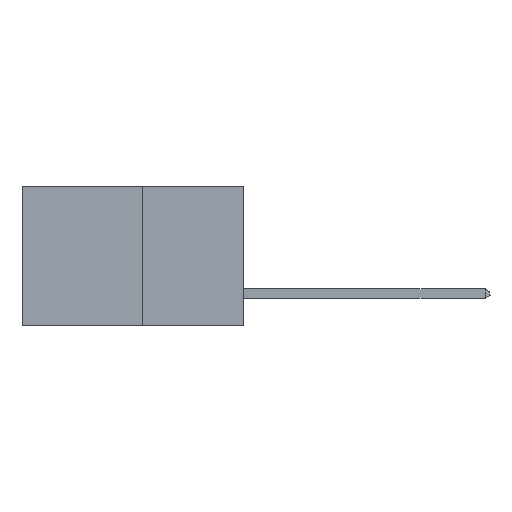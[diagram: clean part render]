
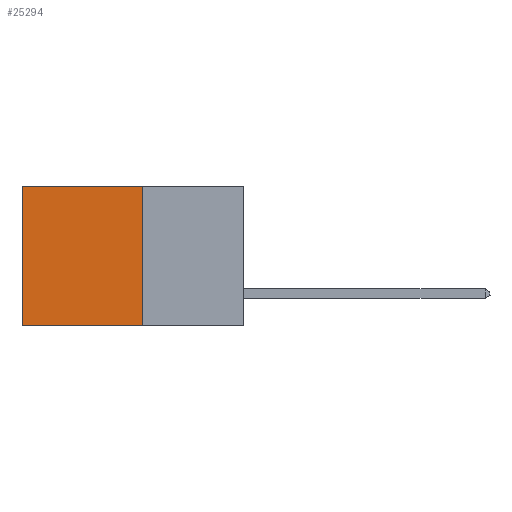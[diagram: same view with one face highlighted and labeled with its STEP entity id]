
A CAD part, left-side view. The second image highlights one B-rep face of the part: STEP entity #25294.
In plain terms, the highlighted planar face has unit normal (-1, 0, 0).
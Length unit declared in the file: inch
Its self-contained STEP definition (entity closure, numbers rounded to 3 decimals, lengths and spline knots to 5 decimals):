
#640 = CARTESIAN_POINT ( 'NONE',  ( 0.277, 0.59, 0. ) ) ;
#789 = DIRECTION ( 'NONE',  ( 0., 1., 0. ) ) ;
#1320 = VERTEX_POINT ( 'NONE', #11204 ) ;
#1961 = CARTESIAN_POINT ( 'NONE',  ( 0.277, 0.27, -0.37 ) ) ;
#2572 = EDGE_CURVE ( 'NONE', #13739, #1320, #28361, .T. ) ;
#3991 = VECTOR ( 'NONE', #12583, 39.37008 ) ;
#4386 = FACE_OUTER_BOUND ( 'NONE', #16905, .T. ) ;
#5601 = ORIENTED_EDGE ( 'NONE', *, *, #12651, .F. ) ;
#6163 = AXIS2_PLACEMENT_3D ( 'NONE', #1961, #22566, #9011 ) ;
#6635 = LINE ( 'NONE', #16857, #12739 ) ;
#6698 = PLANE ( 'NONE',  #6163 ) ;
#9011 = DIRECTION ( 'NONE',  ( 0., 0., -1. ) ) ;
#10261 = VERTEX_POINT ( 'NONE', #640 ) ;
#10298 = CARTESIAN_POINT ( 'NONE',  ( 0.277, 0.59, -0.37 ) ) ;
#10349 = EDGE_CURVE ( 'NONE', #10261, #1320, #22900, .T. ) ;
#10767 = VERTEX_POINT ( 'NONE', #20615 ) ;
#11204 = CARTESIAN_POINT ( 'NONE',  ( 0.277, 0.59, -0.37 ) ) ;
#12583 = DIRECTION ( 'NONE',  ( 0., 0., -1. ) ) ;
#12651 = EDGE_CURVE ( 'NONE', #10767, #13739, #23096, .T. ) ;
#12739 = VECTOR ( 'NONE', #789, 39.37008 ) ;
#13739 = VERTEX_POINT ( 'NONE', #24845 ) ;
#14686 = DIRECTION ( 'NONE',  ( 0., 0., -1. ) ) ;
#16041 = ORIENTED_EDGE ( 'NONE', *, *, #10349, .T. ) ;
#16857 = CARTESIAN_POINT ( 'NONE',  ( 0.277, 0.27, 0. ) ) ;
#16905 = EDGE_LOOP ( 'NONE', ( #16041, #18415, #5601, #23779 ) ) ;
#18415 = ORIENTED_EDGE ( 'NONE', *, *, #2572, .F. ) ;
#19238 = EDGE_CURVE ( 'NONE', #10767, #10261, #6635, .T. ) ;
#20615 = CARTESIAN_POINT ( 'NONE',  ( 0.277, 0.27, 0. ) ) ;
#21403 = CARTESIAN_POINT ( 'NONE',  ( 0.277, 0.27, -0.37 ) ) ;
#22566 = DIRECTION ( 'NONE',  ( 1., 0., 0. ) ) ;
#22900 = LINE ( 'NONE', #10298, #3991 ) ;
#23096 = LINE ( 'NONE', #21403, #23774 ) ;
#23774 = VECTOR ( 'NONE', #14686, 39.37008 ) ;
#23779 = ORIENTED_EDGE ( 'NONE', *, *, #19238, .T. ) ;
#24845 = CARTESIAN_POINT ( 'NONE',  ( 0.277, 0.27, -0.37 ) ) ;
#25294 = ADVANCED_FACE ( 'NONE', ( #4386 ), #6698, .F. ) ;
#26976 = VECTOR ( 'NONE', #28139, 39.37008 ) ;
#28028 = CARTESIAN_POINT ( 'NONE',  ( 0.277, 0.27, -0.37 ) ) ;
#28139 = DIRECTION ( 'NONE',  ( 0., 1., 0. ) ) ;
#28361 = LINE ( 'NONE', #28028, #26976 ) ;
